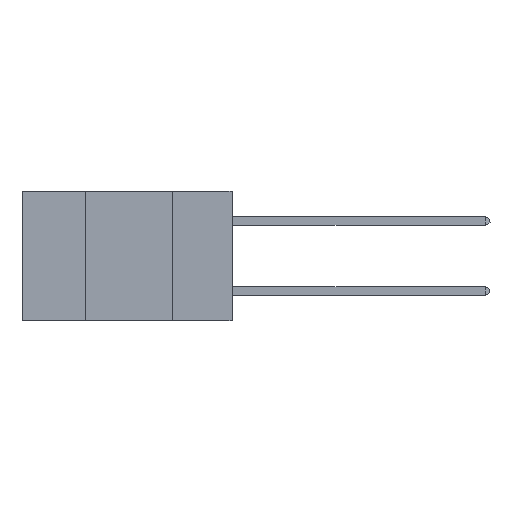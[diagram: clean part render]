
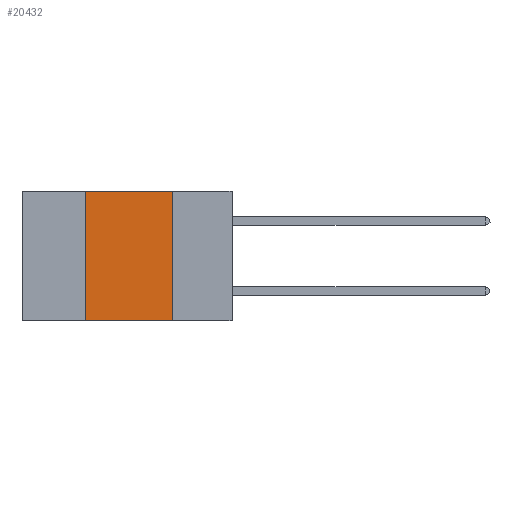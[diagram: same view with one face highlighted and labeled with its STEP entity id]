
A CAD part, left-side view. The second image highlights one B-rep face of the part: STEP entity #20432.
In plain terms, the highlighted planar face has unit normal (-1, 0, 0).
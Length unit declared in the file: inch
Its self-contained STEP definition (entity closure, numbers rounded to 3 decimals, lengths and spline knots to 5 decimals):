
#803 = VERTEX_POINT ( 'NONE', #9691 ) ;
#832 = CARTESIAN_POINT ( 'NONE',  ( 0., 0.6, 0. ) ) ;
#1767 = EDGE_CURVE ( 'NONE', #10316, #11700, #22383, .T. ) ;
#3033 = DIRECTION ( 'NONE',  ( 0., 0., -1. ) ) ;
#3838 = DIRECTION ( 'NONE',  ( 1., 0., 0. ) ) ;
#5049 = LINE ( 'NONE', #26185, #21263 ) ;
#6713 = VECTOR ( 'NONE', #24983, 39.37008 ) ;
#8084 = ORIENTED_EDGE ( 'NONE', *, *, #13249, .F. ) ;
#9691 = CARTESIAN_POINT ( 'NONE',  ( 0., 0.17, 0. ) ) ;
#10316 = VERTEX_POINT ( 'NONE', #30918 ) ;
#11700 = VERTEX_POINT ( 'NONE', #34887 ) ;
#13249 = EDGE_CURVE ( 'NONE', #11700, #803, #20029, .T. ) ;
#13513 = ORIENTED_EDGE ( 'NONE', *, *, #23434, .T. ) ;
#14105 = ORIENTED_EDGE ( 'NONE', *, *, #1767, .F. ) ;
#15006 = EDGE_LOOP ( 'NONE', ( #22904, #8084, #14105, #13513 ) ) ;
#16794 = CARTESIAN_POINT ( 'NONE',  ( 0., 0.42, 0. ) ) ;
#17157 = DIRECTION ( 'NONE',  ( 0., 0., 1. ) ) ;
#20029 = LINE ( 'NONE', #832, #30380 ) ;
#20432 = ADVANCED_FACE ( 'NONE', ( #23168 ), #32777, .F. ) ;
#21263 = VECTOR ( 'NONE', #3033, 39.37008 ) ;
#21876 = AXIS2_PLACEMENT_3D ( 'NONE', #35337, #3838, #32658 ) ;
#22383 = LINE ( 'NONE', #16794, #32751 ) ;
#22810 = CARTESIAN_POINT ( 'NONE',  ( 0., 0.17, -0.37 ) ) ;
#22904 = ORIENTED_EDGE ( 'NONE', *, *, #32060, .F. ) ;
#23168 = FACE_OUTER_BOUND ( 'NONE', #15006, .T. ) ;
#23434 = EDGE_CURVE ( 'NONE', #10316, #24252, #32411, .T. ) ;
#24252 = VERTEX_POINT ( 'NONE', #22810 ) ;
#24983 = DIRECTION ( 'NONE',  ( 0., -1., 0. ) ) ;
#26185 = CARTESIAN_POINT ( 'NONE',  ( 0., 0.17, 0. ) ) ;
#30380 = VECTOR ( 'NONE', #35859, 39.37008 ) ;
#30638 = CARTESIAN_POINT ( 'NONE',  ( 0., 0.6, -0.37 ) ) ;
#30918 = CARTESIAN_POINT ( 'NONE',  ( 0., 0.42, -0.37 ) ) ;
#32060 = EDGE_CURVE ( 'NONE', #803, #24252, #5049, .T. ) ;
#32411 = LINE ( 'NONE', #30638, #6713 ) ;
#32658 = DIRECTION ( 'NONE',  ( 0., 0., -1. ) ) ;
#32751 = VECTOR ( 'NONE', #17157, 39.37008 ) ;
#32777 = PLANE ( 'NONE',  #21876 ) ;
#34887 = CARTESIAN_POINT ( 'NONE',  ( 0., 0.42, 0. ) ) ;
#35337 = CARTESIAN_POINT ( 'NONE',  ( 0., 0.6, 0. ) ) ;
#35859 = DIRECTION ( 'NONE',  ( 0., -1., 0. ) ) ;
